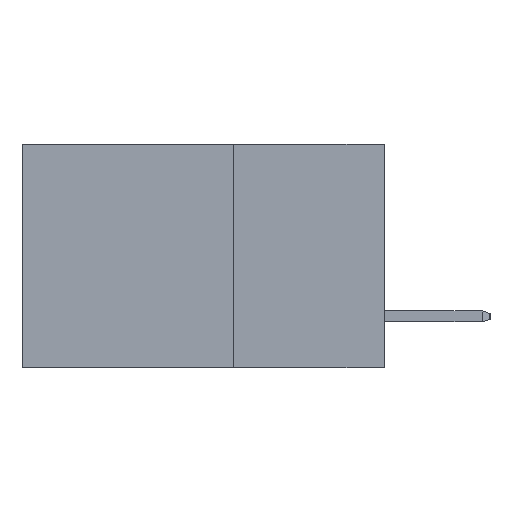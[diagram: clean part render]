
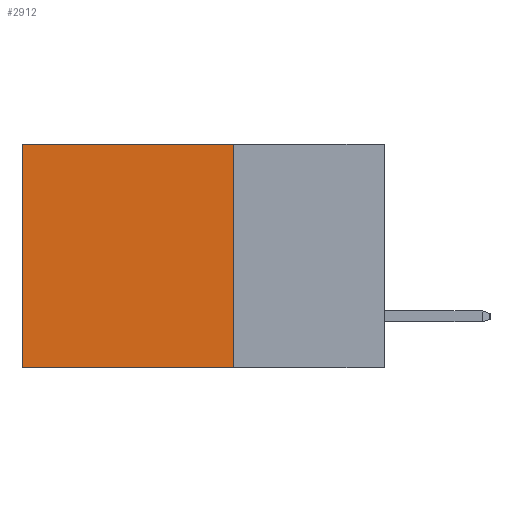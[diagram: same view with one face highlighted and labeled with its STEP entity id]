
A CAD part, left-side view. The second image highlights one B-rep face of the part: STEP entity #2912.
In plain terms, the highlighted planar face has unit normal (-1, 0, 0).
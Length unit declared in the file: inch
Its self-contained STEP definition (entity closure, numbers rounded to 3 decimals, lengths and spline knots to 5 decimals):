
#42 = LINE ( 'NONE', #7403, #4685 ) ;
#113 = ORIENTED_EDGE ( 'NONE', *, *, #209, .F. ) ;
#209 = EDGE_CURVE ( 'NONE', #2951, #4821, #8402, .T. ) ;
#1097 = LINE ( 'NONE', #1876, #3471 ) ;
#1876 = CARTESIAN_POINT ( 'NONE',  ( 0.298, 0.25, -0.37 ) ) ;
#2048 = EDGE_LOOP ( 'NONE', ( #10256, #3121, #113, #7515 ) ) ;
#2455 = DIRECTION ( 'NONE',  ( 0., 0., -1. ) ) ;
#2523 = CARTESIAN_POINT ( 'NONE',  ( 0.298, 0.25, 0. ) ) ;
#2546 = PLANE ( 'NONE',  #5974 ) ;
#2912 = ADVANCED_FACE ( 'NONE', ( #3000 ), #2546, .F. ) ;
#2951 = VERTEX_POINT ( 'NONE', #9811 ) ;
#3000 = FACE_OUTER_BOUND ( 'NONE', #2048, .T. ) ;
#3121 = ORIENTED_EDGE ( 'NONE', *, *, #10731, .F. ) ;
#3471 = VECTOR ( 'NONE', #7809, 39.37008 ) ;
#4151 = VERTEX_POINT ( 'NONE', #9513 ) ;
#4204 = VERTEX_POINT ( 'NONE', #9254 ) ;
#4685 = VECTOR ( 'NONE', #10739, 39.37008 ) ;
#4821 = VERTEX_POINT ( 'NONE', #11054 ) ;
#4847 = VECTOR ( 'NONE', #6657, 39.37008 ) ;
#5974 = AXIS2_PLACEMENT_3D ( 'NONE', #8650, #9754, #9741 ) ;
#6135 = VECTOR ( 'NONE', #2455, 39.37008 ) ;
#6582 = CARTESIAN_POINT ( 'NONE',  ( 0.298, 0.25, 0. ) ) ;
#6657 = DIRECTION ( 'NONE',  ( 0., 1., 0. ) ) ;
#7346 = LINE ( 'NONE', #6582, #4847 ) ;
#7403 = CARTESIAN_POINT ( 'NONE',  ( 0.298, 0.6, 0. ) ) ;
#7515 = ORIENTED_EDGE ( 'NONE', *, *, #7545, .T. ) ;
#7545 = EDGE_CURVE ( 'NONE', #2951, #4204, #7346, .T. ) ;
#7809 = DIRECTION ( 'NONE',  ( 0., 1., 0. ) ) ;
#8402 = LINE ( 'NONE', #2523, #6135 ) ;
#8650 = CARTESIAN_POINT ( 'NONE',  ( 0.298, 0.25, 0. ) ) ;
#9254 = CARTESIAN_POINT ( 'NONE',  ( 0.298, 0.6, 0. ) ) ;
#9499 = EDGE_CURVE ( 'NONE', #4204, #4151, #42, .T. ) ;
#9513 = CARTESIAN_POINT ( 'NONE',  ( 0.298, 0.6, -0.37 ) ) ;
#9741 = DIRECTION ( 'NONE',  ( 0., 0., -1. ) ) ;
#9754 = DIRECTION ( 'NONE',  ( 1., 0., 0. ) ) ;
#9811 = CARTESIAN_POINT ( 'NONE',  ( 0.298, 0.25, 0. ) ) ;
#10256 = ORIENTED_EDGE ( 'NONE', *, *, #9499, .T. ) ;
#10731 = EDGE_CURVE ( 'NONE', #4821, #4151, #1097, .T. ) ;
#10739 = DIRECTION ( 'NONE',  ( 0., 0., -1. ) ) ;
#11054 = CARTESIAN_POINT ( 'NONE',  ( 0.298, 0.25, -0.37 ) ) ;
